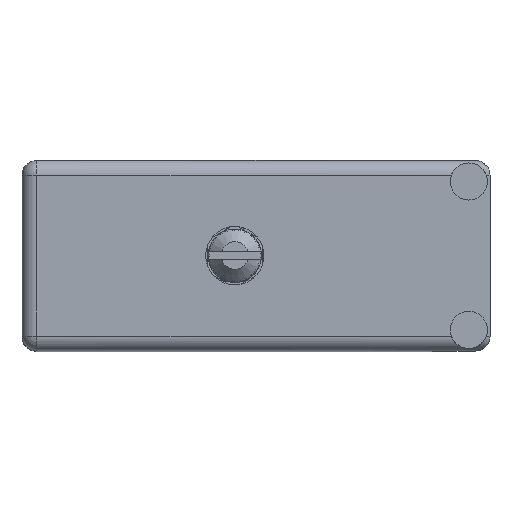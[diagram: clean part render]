
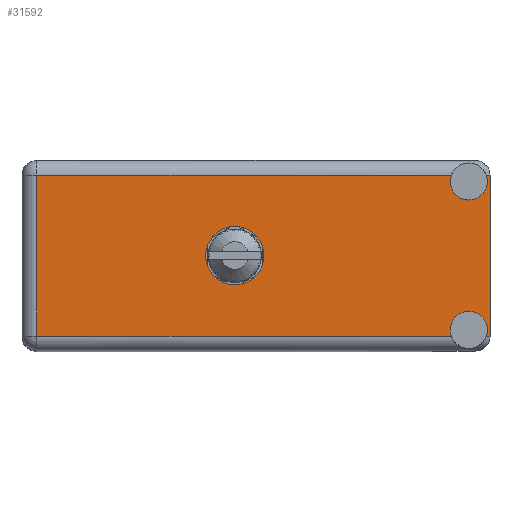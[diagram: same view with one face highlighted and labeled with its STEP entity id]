
A CAD part, top view. The second image highlights one B-rep face of the part: STEP entity #31592.
In plain terms, the highlighted face is planar.
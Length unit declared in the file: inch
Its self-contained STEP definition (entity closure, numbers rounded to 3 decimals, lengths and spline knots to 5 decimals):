
#1654 = DIRECTION ( 'NONE',  ( 0., 1., 0. ) ) ;
#2339 = CARTESIAN_POINT ( 'NONE',  ( 0., 1.466, 0. ) ) ;
#2604 = ORIENTED_EDGE ( 'NONE', *, *, #5936, .F. ) ;
#5864 = ORIENTED_EDGE ( 'NONE', *, *, #78794, .T. ) ;
#5936 = EDGE_CURVE ( 'NONE', #28076, #99504, #94178, .T. ) ;
#6083 = LINE ( 'NONE', #96195, #8630 ) ;
#7117 = CARTESIAN_POINT ( 'NONE',  ( 1.104, 1.466, -0.35 ) ) ;
#8243 = CARTESIAN_POINT ( 'NONE',  ( 1.104, 1.466, -0.2625 ) ) ;
#8630 = VECTOR ( 'NONE', #23412, 39.37008 ) ;
#10238 = CARTESIAN_POINT ( 'NONE',  ( -0.934, 1.466, -0.4495 ) ) ;
#10884 = CIRCLE ( 'NONE', #86933, 0.1375 ) ;
#10949 = AXIS2_PLACEMENT_3D ( 'NONE', #31118, #64262, #72807 ) ;
#11258 = EDGE_LOOP ( 'NONE', ( #91894, #25512, #82947, #72570, #51164, #5864, #81331, #2604, #52141, #73750 ) ) ;
#11573 = VECTOR ( 'NONE', #35322, 39.37008 ) ;
#13855 = EDGE_CURVE ( 'NONE', #65859, #58311, #10884, .T. ) ;
#14396 = DIRECTION ( 'NONE',  ( 0., 0., 1. ) ) ;
#15837 = PLANE ( 'NONE',  #10949 ) ;
#19110 = CARTESIAN_POINT ( 'NONE',  ( -1.004, 1.466, -0.3795 ) ) ;
#19312 = VECTOR ( 'NONE', #27259, 39.37008 ) ;
#19707 = AXIS2_PLACEMENT_3D ( 'NONE', #7117, #64804, #105815 ) ;
#23412 = DIRECTION ( 'NONE',  ( 1., 0., 0. ) ) ;
#24078 = FACE_OUTER_BOUND ( 'NONE', #11258, .T. ) ;
#24353 = LINE ( 'NONE', #76110, #19312 ) ;
#25512 = ORIENTED_EDGE ( 'NONE', *, *, #94874, .F. ) ;
#26159 = VECTOR ( 'NONE', #76478, 39.37008 ) ;
#27132 = EDGE_CURVE ( 'NONE', #75616, #48880, #104020, .T. ) ;
#27259 = DIRECTION ( 'NONE',  ( 1., 0., 0. ) ) ;
#27996 = EDGE_CURVE ( 'NONE', #32827, #84899, #49029, .T. ) ;
#28059 = LINE ( 'NONE', #19110, #93156 ) ;
#28076 = VERTEX_POINT ( 'NONE', #102838 ) ;
#29078 = DIRECTION ( 'NONE',  ( 0., 1., 0. ) ) ;
#30380 = DIRECTION ( 'NONE',  ( 0., 1., 0. ) ) ;
#30700 = CARTESIAN_POINT ( 'NONE',  ( 1.02162, 1.466, 0.3795 ) ) ;
#31118 = CARTESIAN_POINT ( 'NONE',  ( -1.004, 1.466, -0.4495 ) ) ;
#31592 = ADVANCED_FACE ( 'NONE', ( #81283, #24078 ), #15837, .T. ) ;
#32827 = VERTEX_POINT ( 'NONE', #81332 ) ;
#34929 = VERTEX_POINT ( 'NONE', #30700 ) ;
#35322 = DIRECTION ( 'NONE',  ( -1., 0., 0. ) ) ;
#37824 = CARTESIAN_POINT ( 'NONE',  ( 1.104, 1.466, 0.35 ) ) ;
#39267 = ORIENTED_EDGE ( 'NONE', *, *, #88045, .F. ) ;
#39283 = EDGE_CURVE ( 'NONE', #93348, #87408, #81314, .T. ) ;
#42891 = EDGE_LOOP ( 'NONE', ( #39267, #48642 ) ) ;
#43196 = DIRECTION ( 'NONE',  ( 0., 1., 0. ) ) ;
#43257 = EDGE_CURVE ( 'NONE', #28076, #32827, #28059, .T. ) ;
#46019 = EDGE_CURVE ( 'NONE', #99504, #46260, #65936, .T. ) ;
#46120 = CARTESIAN_POINT ( 'NONE',  ( 1.104, 1.466, 0.35 ) ) ;
#46260 = VERTEX_POINT ( 'NONE', #89712 ) ;
#47790 = AXIS2_PLACEMENT_3D ( 'NONE', #92089, #43196, #76404 ) ;
#48642 = ORIENTED_EDGE ( 'NONE', *, *, #13855, .F. ) ;
#48880 = VERTEX_POINT ( 'NONE', #72719 ) ;
#48951 = CIRCLE ( 'NONE', #62226, 0.0875 ) ;
#49029 = LINE ( 'NONE', #10238, #26159 ) ;
#49811 = CARTESIAN_POINT ( 'NONE',  ( 1.204, 1.466, 0.4495 ) ) ;
#51164 = ORIENTED_EDGE ( 'NONE', *, *, #39283, .F. ) ;
#52141 = ORIENTED_EDGE ( 'NONE', *, *, #43257, .T. ) ;
#54114 = AXIS2_PLACEMENT_3D ( 'NONE', #46120, #29078, #95418 ) ;
#57682 = DIRECTION ( 'NONE',  ( 0., 0., 1. ) ) ;
#58311 = VERTEX_POINT ( 'NONE', #78361 ) ;
#59594 = VECTOR ( 'NONE', #57682, 39.37008 ) ;
#59645 = EDGE_CURVE ( 'NONE', #75616, #87408, #6083, .T. ) ;
#61932 = DIRECTION ( 'NONE',  ( 0., 0., 1. ) ) ;
#62226 = AXIS2_PLACEMENT_3D ( 'NONE', #37824, #30380, #14396 ) ;
#64262 = DIRECTION ( 'NONE',  ( 0., 1., 0. ) ) ;
#64804 = DIRECTION ( 'NONE',  ( 0., 1., 0. ) ) ;
#65859 = VERTEX_POINT ( 'NONE', #65911 ) ;
#65911 = CARTESIAN_POINT ( 'NONE',  ( 0., 1.466, -0.1375 ) ) ;
#65936 = CIRCLE ( 'NONE', #101609, 0.0875 ) ;
#68916 = LINE ( 'NONE', #84150, #11573 ) ;
#72570 = ORIENTED_EDGE ( 'NONE', *, *, #59645, .T. ) ;
#72719 = CARTESIAN_POINT ( 'NONE',  ( 1.104, 1.466, 0.2625 ) ) ;
#72807 = DIRECTION ( 'NONE',  ( -1., 0., 0. ) ) ;
#73582 = CARTESIAN_POINT ( 'NONE',  ( -0.934, 1.466, 0.3795 ) ) ;
#73750 = ORIENTED_EDGE ( 'NONE', *, *, #27996, .T. ) ;
#74064 = CARTESIAN_POINT ( 'NONE',  ( 1.204, 1.466, 0.3795 ) ) ;
#75616 = VERTEX_POINT ( 'NONE', #94342 ) ;
#76110 = CARTESIAN_POINT ( 'NONE',  ( 1.204, 1.466, 0.3795 ) ) ;
#76404 = DIRECTION ( 'NONE',  ( 0., 0., 1. ) ) ;
#76478 = DIRECTION ( 'NONE',  ( 0., 0., 1. ) ) ;
#78361 = CARTESIAN_POINT ( 'NONE',  ( 0., 1.466, 0.1375 ) ) ;
#78794 = EDGE_CURVE ( 'NONE', #93348, #46260, #68916, .T. ) ;
#81283 = FACE_BOUND ( 'NONE', #42891, .T. ) ;
#81314 = LINE ( 'NONE', #49811, #59594 ) ;
#81331 = ORIENTED_EDGE ( 'NONE', *, *, #46019, .F. ) ;
#81332 = CARTESIAN_POINT ( 'NONE',  ( -0.934, 1.466, -0.3795 ) ) ;
#82947 = ORIENTED_EDGE ( 'NONE', *, *, #27132, .F. ) ;
#83900 = DIRECTION ( 'NONE',  ( -1., 0., 0. ) ) ;
#84150 = CARTESIAN_POINT ( 'NONE',  ( -1.004, 1.466, -0.3795 ) ) ;
#84899 = VERTEX_POINT ( 'NONE', #73582 ) ;
#85461 = DIRECTION ( 'NONE',  ( 0., 1., 0. ) ) ;
#86933 = AXIS2_PLACEMENT_3D ( 'NONE', #2339, #1654, #91809 ) ;
#87408 = VERTEX_POINT ( 'NONE', #74064 ) ;
#88045 = EDGE_CURVE ( 'NONE', #58311, #65859, #93293, .T. ) ;
#89712 = CARTESIAN_POINT ( 'NONE',  ( 1.18638, 1.466, -0.3795 ) ) ;
#91809 = DIRECTION ( 'NONE',  ( 0., 0., 1. ) ) ;
#91894 = ORIENTED_EDGE ( 'NONE', *, *, #97866, .T. ) ;
#92089 = CARTESIAN_POINT ( 'NONE',  ( 0., 1.466, 0. ) ) ;
#93151 = CARTESIAN_POINT ( 'NONE',  ( 1.204, 1.466, -0.3795 ) ) ;
#93156 = VECTOR ( 'NONE', #83900, 39.37008 ) ;
#93293 = CIRCLE ( 'NONE', #47790, 0.1375 ) ;
#93348 = VERTEX_POINT ( 'NONE', #93151 ) ;
#94178 = CIRCLE ( 'NONE', #19707, 0.0875 ) ;
#94342 = CARTESIAN_POINT ( 'NONE',  ( 1.18638, 1.466, 0.3795 ) ) ;
#94440 = CARTESIAN_POINT ( 'NONE',  ( 1.104, 1.466, -0.35 ) ) ;
#94874 = EDGE_CURVE ( 'NONE', #48880, #34929, #48951, .T. ) ;
#95418 = DIRECTION ( 'NONE',  ( 0., 0., 1. ) ) ;
#96195 = CARTESIAN_POINT ( 'NONE',  ( 1.204, 1.466, 0.3795 ) ) ;
#97866 = EDGE_CURVE ( 'NONE', #84899, #34929, #24353, .T. ) ;
#99504 = VERTEX_POINT ( 'NONE', #8243 ) ;
#101609 = AXIS2_PLACEMENT_3D ( 'NONE', #94440, #85461, #61932 ) ;
#102838 = CARTESIAN_POINT ( 'NONE',  ( 1.02162, 1.466, -0.3795 ) ) ;
#104020 = CIRCLE ( 'NONE', #54114, 0.0875 ) ;
#105815 = DIRECTION ( 'NONE',  ( 0., 0., 1. ) ) ;
